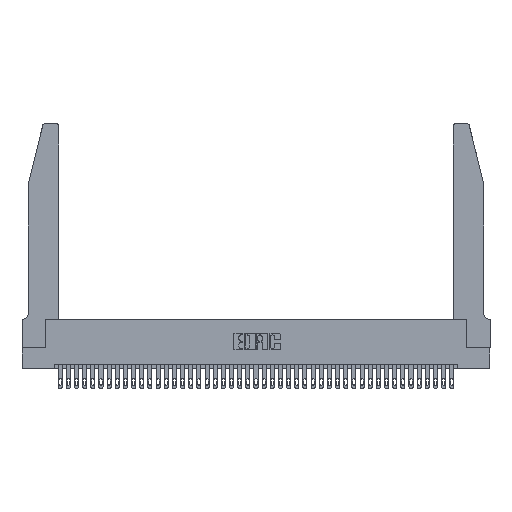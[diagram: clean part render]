
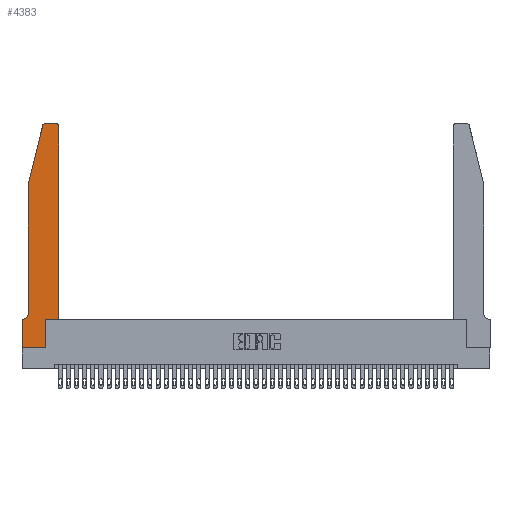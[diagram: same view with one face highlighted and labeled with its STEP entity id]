
A CAD part, top view. The second image highlights one B-rep face of the part: STEP entity #4383.
In plain terms, the highlighted planar face has unit normal (0, 0, 1).
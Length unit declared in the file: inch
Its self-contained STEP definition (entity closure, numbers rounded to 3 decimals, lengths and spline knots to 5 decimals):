
#271 = DIRECTION ( 'NONE',  ( 1., 0., 0. ) ) ;
#592 = CIRCLE ( 'NONE', #18585, 0.03 ) ;
#632 = VERTEX_POINT ( 'NONE', #25604 ) ;
#846 = VECTOR ( 'NONE', #25801, 39.37008 ) ;
#2670 = CARTESIAN_POINT ( 'NONE',  ( 0.0755, 0.35, 0.37 ) ) ;
#3147 = CARTESIAN_POINT ( 'NONE',  ( 0.25487, 2.72718, 0.37 ) ) ;
#3342 = CARTESIAN_POINT ( 'NONE',  ( 0.284, 2.72, 0.37 ) ) ;
#3488 = ORIENTED_EDGE ( 'NONE', *, *, #19358, .T. ) ;
#4238 = DIRECTION ( 'NONE',  ( 1., 0., 0. ) ) ;
#4383 = ADVANCED_FACE ( 'NONE', ( #19004 ), #14934, .T. ) ;
#4470 = VERTEX_POINT ( 'NONE', #7534 ) ;
#6277 = DIRECTION ( 'NONE',  ( -0.239, -0.971, 0. ) ) ;
#6742 = VERTEX_POINT ( 'NONE', #40985 ) ;
#7534 = CARTESIAN_POINT ( 'NONE',  ( 0.4505, 2.72, 0.37 ) ) ;
#7567 = VECTOR ( 'NONE', #22022, 39.37008 ) ;
#8108 = VERTEX_POINT ( 'NONE', #3147 ) ;
#8565 = CARTESIAN_POINT ( 'NONE',  ( 0.284, 2.75, 0.37 ) ) ;
#9603 = LINE ( 'NONE', #12966, #846 ) ;
#9746 = EDGE_CURVE ( 'NONE', #36890, #36664, #12666, .T. ) ;
#10301 = LINE ( 'NONE', #36265, #41408 ) ;
#10318 = LINE ( 'NONE', #30152, #31776 ) ;
#11438 = ORIENTED_EDGE ( 'NONE', *, *, #35901, .T. ) ;
#12666 = LINE ( 'NONE', #23944, #7567 ) ;
#12966 = CARTESIAN_POINT ( 'NONE',  ( 0.4505, 0.35, 0.37 ) ) ;
#13235 = AXIS2_PLACEMENT_3D ( 'NONE', #42148, #26575, #29878 ) ;
#14934 = PLANE ( 'NONE',  #34785 ) ;
#15688 = ORIENTED_EDGE ( 'NONE', *, *, #36225, .T. ) ;
#16522 = EDGE_CURVE ( 'NONE', #8108, #36890, #19374, .T. ) ;
#17169 = VERTEX_POINT ( 'NONE', #30690 ) ;
#17410 = ORIENTED_EDGE ( 'NONE', *, *, #25973, .T. ) ;
#17616 = CARTESIAN_POINT ( 'NONE',  ( 0., 0., 0.37 ) ) ;
#18585 = AXIS2_PLACEMENT_3D ( 'NONE', #3342, #26100, #271 ) ;
#18735 = ORIENTED_EDGE ( 'NONE', *, *, #34721, .T. ) ;
#18779 = ORIENTED_EDGE ( 'NONE', *, *, #9746, .T. ) ;
#19004 = FACE_OUTER_BOUND ( 'NONE', #24149, .T. ) ;
#19358 = EDGE_CURVE ( 'NONE', #20391, #28615, #26789, .T. ) ;
#19374 = LINE ( 'NONE', #30931, #29127 ) ;
#20205 = CARTESIAN_POINT ( 'NONE',  ( 0.2865, 0.35, 0.37 ) ) ;
#20391 = VERTEX_POINT ( 'NONE', #37388 ) ;
#20757 = VERTEX_POINT ( 'NONE', #25520 ) ;
#21212 = LINE ( 'NONE', #24893, #25823 ) ;
#21620 = DIRECTION ( 'NONE',  ( -1., 0., 0. ) ) ;
#22022 = DIRECTION ( 'NONE',  ( 0., -1., 0. ) ) ;
#22510 = DIRECTION ( 'NONE',  ( -1., 0., 0. ) ) ;
#23052 = DIRECTION ( 'NONE',  ( 0., 0., -1. ) ) ;
#23360 = ORIENTED_EDGE ( 'NONE', *, *, #27351, .T. ) ;
#23507 = LINE ( 'NONE', #17616, #26066 ) ;
#23544 = CARTESIAN_POINT ( 'NONE',  ( 0., 0.35, 0.37 ) ) ;
#23885 = DIRECTION ( 'NONE',  ( 1., 0., 0. ) ) ;
#23944 = CARTESIAN_POINT ( 'NONE',  ( 0.0755, 2., 0.37 ) ) ;
#24149 = EDGE_LOOP ( 'NONE', ( #26369, #18735, #24811, #18779, #15688, #34039, #11438, #17410, #3488, #39116, #33752, #23360 ) ) ;
#24811 = ORIENTED_EDGE ( 'NONE', *, *, #16522, .T. ) ;
#24893 = CARTESIAN_POINT ( 'NONE',  ( 0.2605, 2.75, 0.37 ) ) ;
#25222 = VERTEX_POINT ( 'NONE', #8565 ) ;
#25434 = EDGE_CURVE ( 'NONE', #20757, #6742, #38442, .T. ) ;
#25520 = CARTESIAN_POINT ( 'NONE',  ( 0.0055, 0.35, 0.37 ) ) ;
#25604 = CARTESIAN_POINT ( 'NONE',  ( 0.4505, 0.35, 0.37 ) ) ;
#25801 = DIRECTION ( 'NONE',  ( 1., 0., 0. ) ) ;
#25823 = VECTOR ( 'NONE', #21620, 39.37008 ) ;
#25973 = EDGE_CURVE ( 'NONE', #38474, #20391, #10301, .T. ) ;
#26066 = VECTOR ( 'NONE', #39646, 39.37008 ) ;
#26100 = DIRECTION ( 'NONE',  ( 0., 0., 1. ) ) ;
#26208 = CARTESIAN_POINT ( 'NONE',  ( 0., 0., 0.37 ) ) ;
#26369 = ORIENTED_EDGE ( 'NONE', *, *, #38982, .T. ) ;
#26575 = DIRECTION ( 'NONE',  ( 0., 0., 1. ) ) ;
#26789 = LINE ( 'NONE', #20205, #40060 ) ;
#27351 = EDGE_CURVE ( 'NONE', #4470, #17169, #37176, .T. ) ;
#27981 = CARTESIAN_POINT ( 'NONE',  ( 0.2865, 0.35, 0.37 ) ) ;
#28615 = VERTEX_POINT ( 'NONE', #27981 ) ;
#29127 = VECTOR ( 'NONE', #6277, 39.37008 ) ;
#29522 = CARTESIAN_POINT ( 'NONE',  ( 0.0055, 0.42, 0.37 ) ) ;
#29757 = VECTOR ( 'NONE', #38578, 39.37008 ) ;
#29771 = CARTESIAN_POINT ( 'NONE',  ( 0.0755, 0.42, 0.37 ) ) ;
#29878 = DIRECTION ( 'NONE',  ( 1., 0., 0. ) ) ;
#30152 = CARTESIAN_POINT ( 'NONE',  ( 0.4505, 0.35, 0.37 ) ) ;
#30337 = EDGE_CURVE ( 'NONE', #28615, #632, #9603, .T. ) ;
#30690 = CARTESIAN_POINT ( 'NONE',  ( 0.4205, 2.75, 0.37 ) ) ;
#30931 = CARTESIAN_POINT ( 'NONE',  ( 0.0755, 2., 0.37 ) ) ;
#31713 = DIRECTION ( 'NONE',  ( 0., 0., 1. ) ) ;
#31776 = VECTOR ( 'NONE', #40099, 39.37008 ) ;
#33752 = ORIENTED_EDGE ( 'NONE', *, *, #41649, .T. ) ;
#34039 = ORIENTED_EDGE ( 'NONE', *, *, #25434, .T. ) ;
#34542 = AXIS2_PLACEMENT_3D ( 'NONE', #29522, #23052, #22510 ) ;
#34721 = EDGE_CURVE ( 'NONE', #25222, #8108, #592, .T. ) ;
#34785 = AXIS2_PLACEMENT_3D ( 'NONE', #23544, #31713, #23885 ) ;
#35901 = EDGE_CURVE ( 'NONE', #6742, #38474, #23507, .T. ) ;
#36225 = EDGE_CURVE ( 'NONE', #36664, #20757, #41879, .T. ) ;
#36265 = CARTESIAN_POINT ( 'NONE',  ( 0., 0., 0.37 ) ) ;
#36664 = VERTEX_POINT ( 'NONE', #29771 ) ;
#36890 = VERTEX_POINT ( 'NONE', #40999 ) ;
#37176 = CIRCLE ( 'NONE', #13235, 0.03 ) ;
#37388 = CARTESIAN_POINT ( 'NONE',  ( 0.2865, 0., 0.37 ) ) ;
#38442 = LINE ( 'NONE', #2670, #29757 ) ;
#38474 = VERTEX_POINT ( 'NONE', #26208 ) ;
#38578 = DIRECTION ( 'NONE',  ( -1., 0., 0. ) ) ;
#38982 = EDGE_CURVE ( 'NONE', #17169, #25222, #21212, .T. ) ;
#39116 = ORIENTED_EDGE ( 'NONE', *, *, #30337, .T. ) ;
#39633 = DIRECTION ( 'NONE',  ( 0., 1., 0. ) ) ;
#39646 = DIRECTION ( 'NONE',  ( 0., -1., 0. ) ) ;
#40060 = VECTOR ( 'NONE', #39633, 39.37008 ) ;
#40099 = DIRECTION ( 'NONE',  ( 0., 1., 0. ) ) ;
#40985 = CARTESIAN_POINT ( 'NONE',  ( 0., 0.35, 0.37 ) ) ;
#40999 = CARTESIAN_POINT ( 'NONE',  ( 0.0755, 2., 0.37 ) ) ;
#41408 = VECTOR ( 'NONE', #4238, 39.37008 ) ;
#41649 = EDGE_CURVE ( 'NONE', #632, #4470, #10318, .T. ) ;
#41879 = CIRCLE ( 'NONE', #34542, 0.07 ) ;
#42148 = CARTESIAN_POINT ( 'NONE',  ( 0.4205, 2.72, 0.37 ) ) ;
